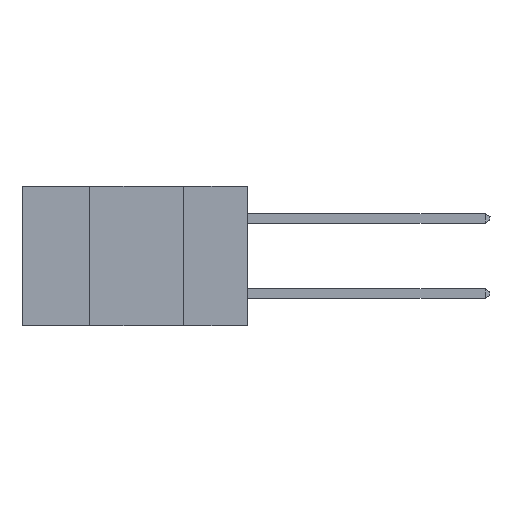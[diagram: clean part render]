
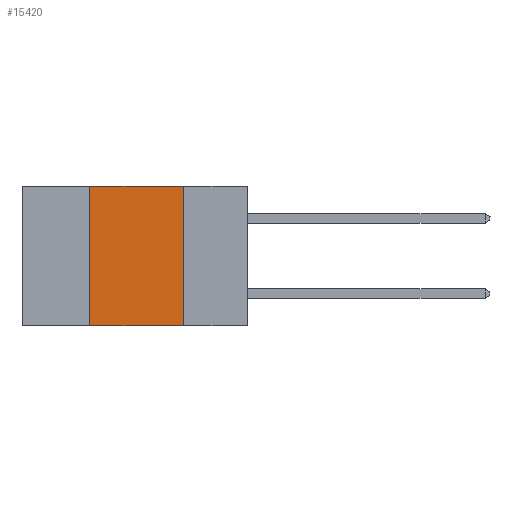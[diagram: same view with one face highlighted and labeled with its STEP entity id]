
A CAD part, left-side view. The second image highlights one B-rep face of the part: STEP entity #15420.
In plain terms, the highlighted planar face has unit normal (-1, 0, 0).
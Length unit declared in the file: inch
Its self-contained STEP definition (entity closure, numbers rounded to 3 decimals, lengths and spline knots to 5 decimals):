
#371 = LINE ( 'NONE', #23207, #6641 ) ;
#3033 = VERTEX_POINT ( 'NONE', #30092 ) ;
#3510 = CARTESIAN_POINT ( 'NONE',  ( 0., 0.42, 0. ) ) ;
#4891 = ORIENTED_EDGE ( 'NONE', *, *, #19444, .F. ) ;
#6220 = DIRECTION ( 'NONE',  ( 0., 0., 1. ) ) ;
#6641 = VECTOR ( 'NONE', #10175, 39.37008 ) ;
#8097 = ORIENTED_EDGE ( 'NONE', *, *, #8849, .F. ) ;
#8273 = LINE ( 'NONE', #3510, #21419 ) ;
#8849 = EDGE_CURVE ( 'NONE', #23713, #17647, #8273, .T. ) ;
#9430 = ORIENTED_EDGE ( 'NONE', *, *, #25136, .T. ) ;
#9652 = CARTESIAN_POINT ( 'NONE',  ( 0., 0.17, -0.37 ) ) ;
#10042 = CARTESIAN_POINT ( 'NONE',  ( 0., 0.6, 0. ) ) ;
#10175 = DIRECTION ( 'NONE',  ( 0., 0., -1. ) ) ;
#10311 = VECTOR ( 'NONE', #30549, 39.37008 ) ;
#10927 = AXIS2_PLACEMENT_3D ( 'NONE', #20473, #30891, #15344 ) ;
#15344 = DIRECTION ( 'NONE',  ( 0., 0., -1. ) ) ;
#15420 = ADVANCED_FACE ( 'NONE', ( #18488 ), #28272, .F. ) ;
#17070 = LINE ( 'NONE', #10042, #23950 ) ;
#17647 = VERTEX_POINT ( 'NONE', #23969 ) ;
#18037 = EDGE_CURVE ( 'NONE', #17647, #3033, #17070, .T. ) ;
#18488 = FACE_OUTER_BOUND ( 'NONE', #26650, .T. ) ;
#19444 = EDGE_CURVE ( 'NONE', #3033, #23408, #371, .T. ) ;
#20473 = CARTESIAN_POINT ( 'NONE',  ( 0., 0.6, 0. ) ) ;
#21419 = VECTOR ( 'NONE', #6220, 39.37008 ) ;
#21667 = CARTESIAN_POINT ( 'NONE',  ( 0., 0.42, -0.37 ) ) ;
#23064 = ORIENTED_EDGE ( 'NONE', *, *, #18037, .F. ) ;
#23207 = CARTESIAN_POINT ( 'NONE',  ( 0., 0.17, 0. ) ) ;
#23408 = VERTEX_POINT ( 'NONE', #9652 ) ;
#23713 = VERTEX_POINT ( 'NONE', #21667 ) ;
#23950 = VECTOR ( 'NONE', #28274, 39.37008 ) ;
#23969 = CARTESIAN_POINT ( 'NONE',  ( 0., 0.42, 0. ) ) ;
#24220 = LINE ( 'NONE', #27947, #10311 ) ;
#25136 = EDGE_CURVE ( 'NONE', #23713, #23408, #24220, .T. ) ;
#26650 = EDGE_LOOP ( 'NONE', ( #4891, #23064, #8097, #9430 ) ) ;
#27947 = CARTESIAN_POINT ( 'NONE',  ( 0., 0.6, -0.37 ) ) ;
#28272 = PLANE ( 'NONE',  #10927 ) ;
#28274 = DIRECTION ( 'NONE',  ( 0., -1., 0. ) ) ;
#30092 = CARTESIAN_POINT ( 'NONE',  ( 0., 0.17, 0. ) ) ;
#30549 = DIRECTION ( 'NONE',  ( 0., -1., 0. ) ) ;
#30891 = DIRECTION ( 'NONE',  ( 1., 0., 0. ) ) ;
